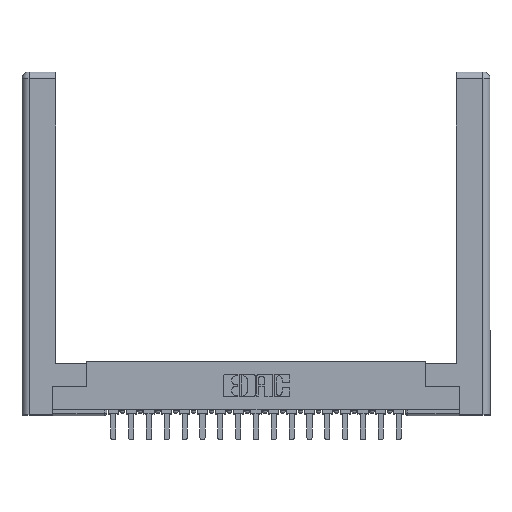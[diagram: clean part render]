
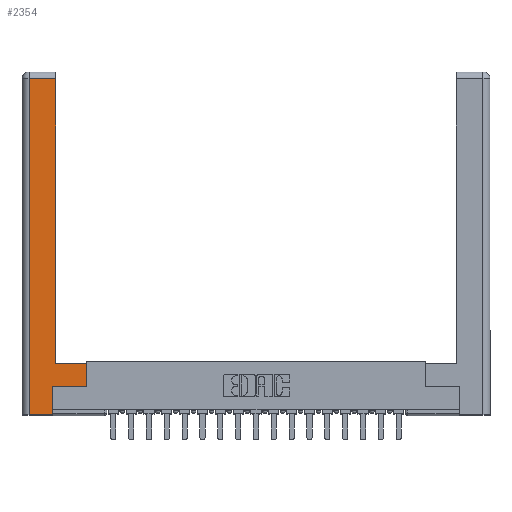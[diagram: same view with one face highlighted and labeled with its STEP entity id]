
A CAD part, top view. The second image highlights one B-rep face of the part: STEP entity #2354.
In plain terms, the highlighted planar face has unit normal (0, 0, 1).
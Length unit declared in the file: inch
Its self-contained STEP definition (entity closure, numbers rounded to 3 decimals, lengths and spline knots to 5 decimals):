
#291 = VECTOR ( 'NONE', #7196, 39.37008 ) ;
#325 = ORIENTED_EDGE ( 'NONE', *, *, #15795, .T. ) ;
#344 = ORIENTED_EDGE ( 'NONE', *, *, #3021, .T. ) ;
#476 = VERTEX_POINT ( 'NONE', #7557 ) ;
#1220 = CARTESIAN_POINT ( 'NONE',  ( 0.295, 3., 0. ) ) ;
#1318 = DIRECTION ( 'NONE',  ( 1., 0., 0. ) ) ;
#1404 = LINE ( 'NONE', #1607, #12060 ) ;
#1607 = CARTESIAN_POINT ( 'NONE',  ( 0.565, 0.245, 0. ) ) ;
#1652 = VERTEX_POINT ( 'NONE', #10917 ) ;
#2354 = ADVANCED_FACE ( 'NONE', ( #14837 ), #17479, .F. ) ;
#2549 = ORIENTED_EDGE ( 'NONE', *, *, #15889, .T. ) ;
#2654 = VECTOR ( 'NONE', #16208, 39.37008 ) ;
#2756 = CARTESIAN_POINT ( 'NONE',  ( 0.565, 0.245, 0. ) ) ;
#3021 = EDGE_CURVE ( 'NONE', #1652, #11263, #15820, .T. ) ;
#3123 = CARTESIAN_POINT ( 'NONE',  ( 0.295, 2.94, 0. ) ) ;
#3617 = CARTESIAN_POINT ( 'NONE',  ( 0.0615, 0., 0. ) ) ;
#3701 = CARTESIAN_POINT ( 'NONE',  ( 0.265, 0., 0. ) ) ;
#4440 = DIRECTION ( 'NONE',  ( 0., 1., 0. ) ) ;
#5010 = DIRECTION ( 'NONE',  ( 0., 1., 0. ) ) ;
#5508 = CARTESIAN_POINT ( 'NONE',  ( 0.0615, 2.94, 0. ) ) ;
#5748 = VECTOR ( 'NONE', #16276, 39.37008 ) ;
#5930 = VECTOR ( 'NONE', #14596, 39.37008 ) ;
#5968 = ORIENTED_EDGE ( 'NONE', *, *, #17715, .T. ) ;
#6189 = EDGE_LOOP ( 'NONE', ( #7089, #11772, #344, #325, #18274, #2549, #12651, #5968 ) ) ;
#6311 = VERTEX_POINT ( 'NONE', #3701 ) ;
#6669 = VERTEX_POINT ( 'NONE', #2756 ) ;
#7089 = ORIENTED_EDGE ( 'NONE', *, *, #18123, .T. ) ;
#7196 = DIRECTION ( 'NONE',  ( -1., 0., 0. ) ) ;
#7514 = LINE ( 'NONE', #12980, #13591 ) ;
#7557 = CARTESIAN_POINT ( 'NONE',  ( 0.295, 0.45, 0. ) ) ;
#7631 = CARTESIAN_POINT ( 'NONE',  ( 0.565, 0.45, 0. ) ) ;
#7986 = DIRECTION ( 'NONE',  ( 0., 0., -1. ) ) ;
#8731 = VECTOR ( 'NONE', #1318, 39.37008 ) ;
#8939 = VECTOR ( 'NONE', #4440, 39.37008 ) ;
#9384 = CARTESIAN_POINT ( 'NONE',  ( 0.265, 0., 0. ) ) ;
#10862 = AXIS2_PLACEMENT_3D ( 'NONE', #20672, #7986, #19301 ) ;
#10917 = CARTESIAN_POINT ( 'NONE',  ( 0.0615, 2.94, 0. ) ) ;
#11263 = VERTEX_POINT ( 'NONE', #3617 ) ;
#11583 = CARTESIAN_POINT ( 'NONE',  ( 0.0615, 0., 0. ) ) ;
#11772 = ORIENTED_EDGE ( 'NONE', *, *, #12097, .T. ) ;
#12052 = CARTESIAN_POINT ( 'NONE',  ( 0.265, 0.245, 0. ) ) ;
#12060 = VECTOR ( 'NONE', #20935, 39.37008 ) ;
#12097 = EDGE_CURVE ( 'NONE', #15020, #1652, #13278, .T. ) ;
#12651 = ORIENTED_EDGE ( 'NONE', *, *, #16063, .T. ) ;
#12980 = CARTESIAN_POINT ( 'NONE',  ( 0.265, 0.245, 0. ) ) ;
#13227 = CARTESIAN_POINT ( 'NONE',  ( 0.295, 0.45, 0. ) ) ;
#13278 = LINE ( 'NONE', #5508, #291 ) ;
#13591 = VECTOR ( 'NONE', #5010, 39.37008 ) ;
#14596 = DIRECTION ( 'NONE',  ( 0., -1., 0. ) ) ;
#14672 = CARTESIAN_POINT ( 'NONE',  ( 0.565, 0.45, 0. ) ) ;
#14837 = FACE_OUTER_BOUND ( 'NONE', #6189, .T. ) ;
#15020 = VERTEX_POINT ( 'NONE', #3123 ) ;
#15571 = LINE ( 'NONE', #1220, #8939 ) ;
#15795 = EDGE_CURVE ( 'NONE', #11263, #6311, #18635, .T. ) ;
#15820 = LINE ( 'NONE', #11583, #5930 ) ;
#15889 = EDGE_CURVE ( 'NONE', #19781, #6669, #1404, .T. ) ;
#16063 = EDGE_CURVE ( 'NONE', #6669, #17620, #19128, .T. ) ;
#16208 = DIRECTION ( 'NONE',  ( -1., 0., 0. ) ) ;
#16276 = DIRECTION ( 'NONE',  ( 0., 1., 0. ) ) ;
#16596 = EDGE_CURVE ( 'NONE', #6311, #19781, #7514, .T. ) ;
#17479 = PLANE ( 'NONE',  #10862 ) ;
#17620 = VERTEX_POINT ( 'NONE', #7631 ) ;
#17715 = EDGE_CURVE ( 'NONE', #17620, #476, #18588, .T. ) ;
#18123 = EDGE_CURVE ( 'NONE', #476, #15020, #15571, .T. ) ;
#18274 = ORIENTED_EDGE ( 'NONE', *, *, #16596, .T. ) ;
#18588 = LINE ( 'NONE', #13227, #2654 ) ;
#18635 = LINE ( 'NONE', #9384, #8731 ) ;
#19128 = LINE ( 'NONE', #14672, #5748 ) ;
#19301 = DIRECTION ( 'NONE',  ( -1., 0., 0. ) ) ;
#19781 = VERTEX_POINT ( 'NONE', #12052 ) ;
#20672 = CARTESIAN_POINT ( 'NONE',  ( 0., 0., 0. ) ) ;
#20935 = DIRECTION ( 'NONE',  ( 1., 0., 0. ) ) ;
